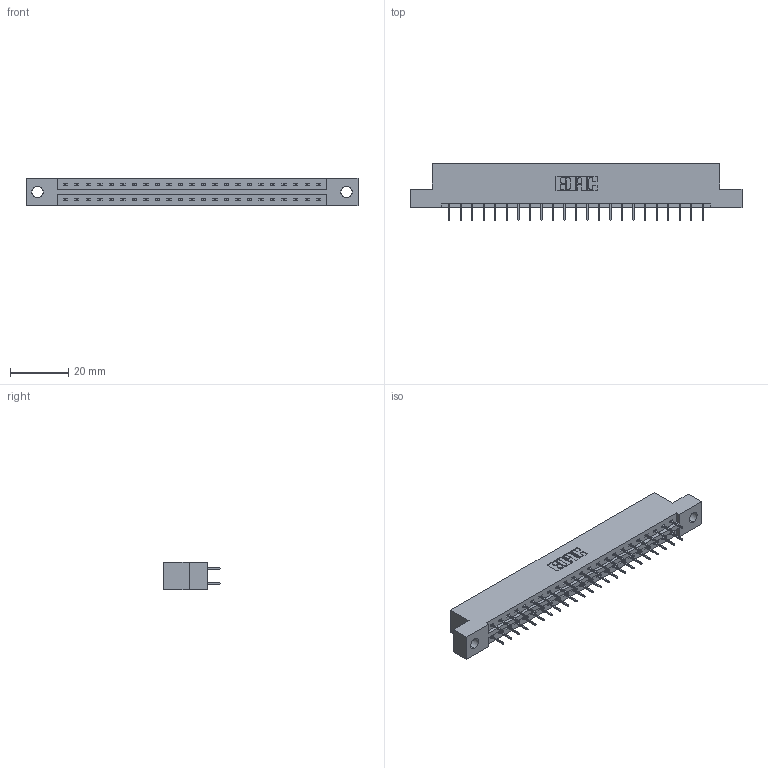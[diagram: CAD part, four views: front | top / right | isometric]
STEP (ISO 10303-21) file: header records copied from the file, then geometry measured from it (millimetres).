
FILE_DESCRIPTION (( 'STEP AP203' ), '1' );
FILE_NAME ('337-046-524-204.STEP', '2018-08-09T07:13:45', ( '' ), ( '' ), 'SwSTEP 2.0', 'SolidWorks 2016', '' );
FILE_SCHEMA (( 'CONFIG_CONTROL_DESIGN' ));
Length unit declared in the file: inch
Products named in the file (3): 337-046-524-204; 337 Part_Flush Mounting Lugs - 0.156 Dia-TH; 345-292-001_345-293-124
Assembly tree (47 placements, depth 2):
  337-046-524-204
    337 Part_Flush Mounting Lugs - 0.156 Dia-TH
    345-292-001_345-293-124  x46
Bounding box: 114.15 x 19.69 x 9.4 mm (x, y, z)
Volume: 11619.4 mm3; surface area: 12533 mm2
Topology: 47 solids, 47 shells, 2782 faces, 7901 edges, 5082 vertices
Faces by surface type: plane 2094, cylinder 688
Entity records: 20367 total; most frequent: CARTESIAN_POINT 3446, ORIENTED_EDGE 3382, DIRECTION 2967, EDGE_CURVE 1691, VECTOR 1567, LINE 1567, VERTEX_POINT 1122, AXIS2_PLACEMENT_3D 700
